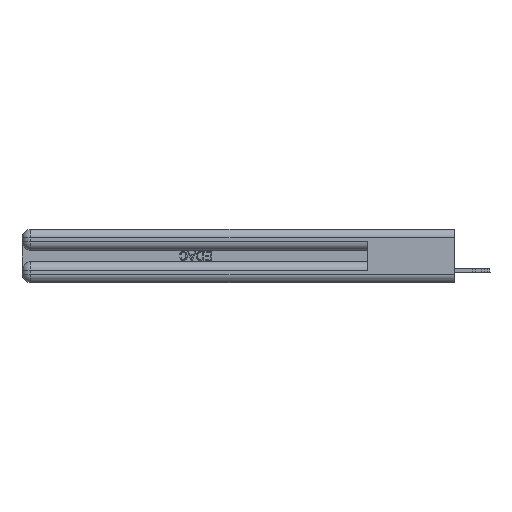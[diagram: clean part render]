
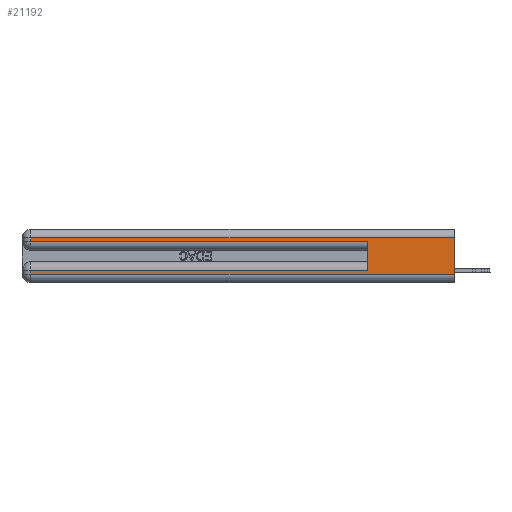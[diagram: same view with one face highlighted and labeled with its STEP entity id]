
A CAD part, left-side view. The second image highlights one B-rep face of the part: STEP entity #21192.
In plain terms, the highlighted planar face has unit normal (-1, 0, 0).
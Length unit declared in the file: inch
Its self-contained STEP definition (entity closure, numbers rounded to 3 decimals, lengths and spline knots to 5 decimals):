
#222 = CARTESIAN_POINT ( 'NONE',  ( 0., 0., 0.06 ) ) ;
#637 = CARTESIAN_POINT ( 'NONE',  ( 0., 0., 0.31 ) ) ;
#1155 = ORIENTED_EDGE ( 'NONE', *, *, #32384, .T. ) ;
#1254 = LINE ( 'NONE', #4661, #16271 ) ;
#1269 = EDGE_LOOP ( 'NONE', ( #32107, #24207, #1155, #10421, #14439, #24302, #3723, #13588 ) ) ;
#1527 = CARTESIAN_POINT ( 'NONE',  ( 0., 2.94, 0.285 ) ) ;
#1561 = VERTEX_POINT ( 'NONE', #6530 ) ;
#2162 = DIRECTION ( 'NONE',  ( 1., 0., 0. ) ) ;
#2391 = EDGE_CURVE ( 'NONE', #11567, #41191, #14847, .T. ) ;
#3415 = FACE_OUTER_BOUND ( 'NONE', #1269, .T. ) ;
#3723 = ORIENTED_EDGE ( 'NONE', *, *, #18802, .T. ) ;
#4064 = VECTOR ( 'NONE', #35744, 39.37008 ) ;
#4583 = VECTOR ( 'NONE', #40045, 39.37008 ) ;
#4661 = CARTESIAN_POINT ( 'NONE',  ( 0., 2.94, 0.37 ) ) ;
#4945 = DIRECTION ( 'NONE',  ( 0., 0., 1. ) ) ;
#5147 = LINE ( 'NONE', #38686, #4064 ) ;
#5468 = PLANE ( 'NONE',  #25109 ) ;
#5655 = DIRECTION ( 'NONE',  ( 0., 0., -1. ) ) ;
#6530 = CARTESIAN_POINT ( 'NONE',  ( 0., 2.94, 0.31 ) ) ;
#7897 = DIRECTION ( 'NONE',  ( 0., 1., 0. ) ) ;
#8926 = CARTESIAN_POINT ( 'NONE',  ( 0., 0.6, 0.145 ) ) ;
#9031 = CARTESIAN_POINT ( 'NONE',  ( 0., 2.94, 0.085 ) ) ;
#10109 = CARTESIAN_POINT ( 'NONE',  ( 0., 0.6, 0.285 ) ) ;
#10421 = ORIENTED_EDGE ( 'NONE', *, *, #19763, .T. ) ;
#10915 = CARTESIAN_POINT ( 'NONE',  ( 0., 0., 0.06 ) ) ;
#11567 = VERTEX_POINT ( 'NONE', #637 ) ;
#11930 = DIRECTION ( 'NONE',  ( 0., 0., -1. ) ) ;
#13588 = ORIENTED_EDGE ( 'NONE', *, *, #23041, .T. ) ;
#13757 = EDGE_CURVE ( 'NONE', #17282, #40852, #20014, .T. ) ;
#14087 = CARTESIAN_POINT ( 'NONE',  ( 0., 2.94, 0.06 ) ) ;
#14439 = ORIENTED_EDGE ( 'NONE', *, *, #28035, .F. ) ;
#14847 = LINE ( 'NONE', #35412, #21757 ) ;
#16271 = VECTOR ( 'NONE', #11930, 39.37008 ) ;
#17282 = VERTEX_POINT ( 'NONE', #30213 ) ;
#18688 = LINE ( 'NONE', #10915, #30914 ) ;
#18802 = EDGE_CURVE ( 'NONE', #40852, #24738, #25501, .T. ) ;
#19518 = LINE ( 'NONE', #23435, #4583 ) ;
#19763 = EDGE_CURVE ( 'NONE', #27410, #24157, #5147, .T. ) ;
#20014 = LINE ( 'NONE', #34571, #42342 ) ;
#21192 = ADVANCED_FACE ( 'NONE', ( #3415 ), #5468, .F. ) ;
#21757 = VECTOR ( 'NONE', #38804, 39.37008 ) ;
#23041 = EDGE_CURVE ( 'NONE', #24738, #41191, #18688, .T. ) ;
#23435 = CARTESIAN_POINT ( 'NONE',  ( 0., 0., 0.31 ) ) ;
#23593 = VECTOR ( 'NONE', #4945, 39.37008 ) ;
#24157 = VERTEX_POINT ( 'NONE', #10109 ) ;
#24207 = ORIENTED_EDGE ( 'NONE', *, *, #31100, .T. ) ;
#24302 = ORIENTED_EDGE ( 'NONE', *, *, #13757, .T. ) ;
#24738 = VERTEX_POINT ( 'NONE', #14087 ) ;
#25109 = AXIS2_PLACEMENT_3D ( 'NONE', #32402, #2162, #26028 ) ;
#25501 = LINE ( 'NONE', #26998, #26571 ) ;
#26028 = DIRECTION ( 'NONE',  ( 0., 0., -1. ) ) ;
#26571 = VECTOR ( 'NONE', #5655, 39.37008 ) ;
#26998 = CARTESIAN_POINT ( 'NONE',  ( 0., 2.94, 0.37 ) ) ;
#27410 = VERTEX_POINT ( 'NONE', #1527 ) ;
#28035 = EDGE_CURVE ( 'NONE', #17282, #24157, #39498, .T. ) ;
#30213 = CARTESIAN_POINT ( 'NONE',  ( 0., 0.6, 0.085 ) ) ;
#30914 = VECTOR ( 'NONE', #38136, 39.37008 ) ;
#31100 = EDGE_CURVE ( 'NONE', #11567, #1561, #19518, .T. ) ;
#32107 = ORIENTED_EDGE ( 'NONE', *, *, #2391, .F. ) ;
#32384 = EDGE_CURVE ( 'NONE', #1561, #27410, #1254, .T. ) ;
#32402 = CARTESIAN_POINT ( 'NONE',  ( 0., 0., 0.37 ) ) ;
#34571 = CARTESIAN_POINT ( 'NONE',  ( 0., 0., 0.085 ) ) ;
#35412 = CARTESIAN_POINT ( 'NONE',  ( 0., 0., 0.37 ) ) ;
#35744 = DIRECTION ( 'NONE',  ( 0., -1., 0. ) ) ;
#38136 = DIRECTION ( 'NONE',  ( 0., -1., 0. ) ) ;
#38686 = CARTESIAN_POINT ( 'NONE',  ( 0., 0., 0.285 ) ) ;
#38804 = DIRECTION ( 'NONE',  ( 0., 0., -1. ) ) ;
#39498 = LINE ( 'NONE', #8926, #23593 ) ;
#40045 = DIRECTION ( 'NONE',  ( 0., 1., 0. ) ) ;
#40852 = VERTEX_POINT ( 'NONE', #9031 ) ;
#41191 = VERTEX_POINT ( 'NONE', #222 ) ;
#42342 = VECTOR ( 'NONE', #7897, 39.37008 ) ;
